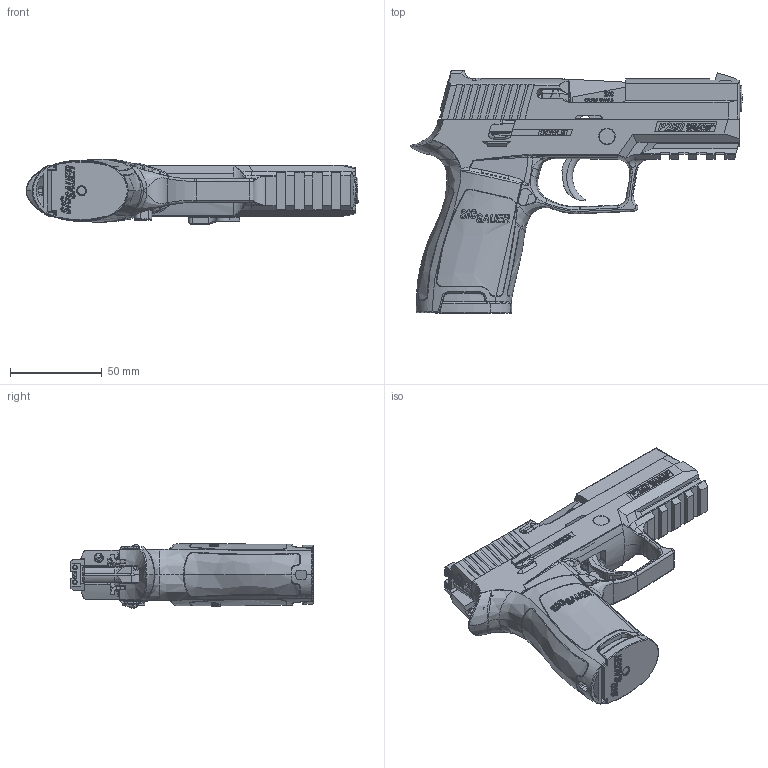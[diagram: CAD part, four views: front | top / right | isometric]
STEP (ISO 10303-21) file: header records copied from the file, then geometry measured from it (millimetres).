
FILE_DESCRIPTION (( 'STEP AP214' ), '1' );
FILE_NAME ('Sig_P250_Complete.STEP', '2014-07-30T19:43:25', ( 'WarFairy' ), ( '' ), 'SwSTEP 2.0', 'SolidWorks 2013', '' );
FILE_SCHEMA (( 'AUTOMOTIVE_DESIGN' ));
Length unit declared in the file: millimetre
Products named in the file (37): Magazine Release Spring; Part31_1; Magazine Insert; Magazine Tube - Copy; Magazine Floorplate; Hammer Pivot Pin; Magazine Catch; Polymer v5 latest backup; Magazine Catch Stop; Trigger; Large Mainspring; Trigger Bar; Hammer; Takedown Lever; Hammer Strut Pin; Takedown Lever O-Ring; Front Sight; Spring Pin; Front Extractor Spring Guide; Small Mainspring; Frame; Slide Catch Lever; Firing Pin; Slide Catch Lever Pin; Firing Pin Spring; Safety Locking Spring; Extractor; Safety Lock; Extractor Spring; Safety Lever; Barrel; Recoil Spring; Slide_1; Recoil Spring Guide; Rear Sight; Sig_P250_Complete; Rear Extractor Spring Guide
Assembly tree (36 placements, depth 2):
  Sig_P250_Complete
    Slide_1
    Barrel
    Extractor Spring
    Extractor
    Firing Pin Spring
    Firing Pin
    Frame
    Front Extractor Spring Guide
    Front Sight
    Hammer Strut Pin
    Hammer
    Large Mainspring
    Magazine Catch Stop
    Magazine Catch
    Magazine Floorplate
    Magazine Insert
    Magazine Release Spring
    Rear Extractor Spring Guide
    Rear Sight
    Recoil Spring Guide
    Recoil Spring
    Safety Lever
    Safety Lock
    Safety Locking Spring
    Slide Catch Lever Pin
    Slide Catch Lever
    Small Mainspring
    Spring Pin
    Takedown Lever O-Ring
    Takedown Lever
    Trigger Bar
    Trigger
    Polymer v5 latest backup
    Hammer Pivot Pin
    Magazine Tube - Copy
    Part31_1
Bounding box: 181.42 x 132.31 x 35.8 mm (x, y, z)
Volume: 161787.6 mm3; surface area: 141326.8 mm2
Topology: 36 solids, 36 shells, 5196 faces, 14221 edges, 9234 vertices
Faces by surface type: plane 2495, bspline 1425, cylinder 1058, torus 158, cone 39, sphere 21
Entity records: 237246 total; most frequent: CARTESIAN_POINT 114985, ORIENTED_EDGE 28362, DIRECTION 19243, EDGE_CURVE 14181, VERTEX_POINT 9230, VECTOR 8045, LINE 8045, AXIS2_PLACEMENT_3D 5599
